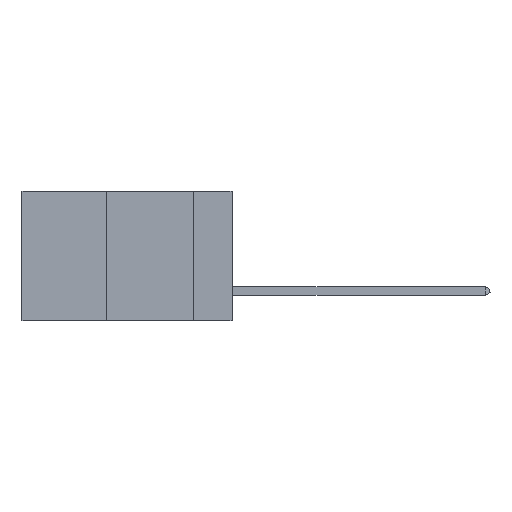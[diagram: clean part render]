
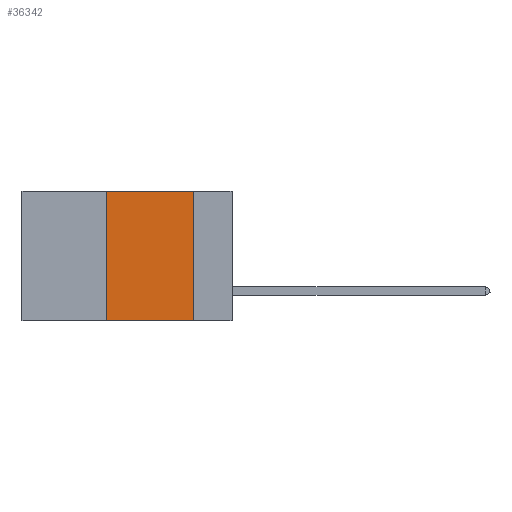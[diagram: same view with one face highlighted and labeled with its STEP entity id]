
A CAD part, left-side view. The second image highlights one B-rep face of the part: STEP entity #36342.
In plain terms, the highlighted planar face has unit normal (-1, 0, 0).
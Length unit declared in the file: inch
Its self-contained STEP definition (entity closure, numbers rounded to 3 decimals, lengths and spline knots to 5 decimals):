
#472 = CARTESIAN_POINT ( 'NONE',  ( 0., 0.36, -0.37 ) ) ;
#2015 = DIRECTION ( 'NONE',  ( 0., -1., 0. ) ) ;
#4391 = ORIENTED_EDGE ( 'NONE', *, *, #30688, .F. ) ;
#5009 = CARTESIAN_POINT ( 'NONE',  ( 0., 0.36, 0. ) ) ;
#8426 = DIRECTION ( 'NONE',  ( 0., 0., 1. ) ) ;
#9119 = ORIENTED_EDGE ( 'NONE', *, *, #25956, .F. ) ;
#10584 = LINE ( 'NONE', #36813, #33721 ) ;
#11051 = CARTESIAN_POINT ( 'NONE',  ( 0., 0.6, 0. ) ) ;
#13673 = AXIS2_PLACEMENT_3D ( 'NONE', #26257, #32345, #29391 ) ;
#14157 = VERTEX_POINT ( 'NONE', #36284 ) ;
#18818 = EDGE_CURVE ( 'NONE', #14157, #27627, #10584, .T. ) ;
#19027 = DIRECTION ( 'NONE',  ( 0., -1., 0. ) ) ;
#19189 = ORIENTED_EDGE ( 'NONE', *, *, #20875, .T. ) ;
#19278 = ORIENTED_EDGE ( 'NONE', *, *, #18818, .F. ) ;
#20875 = EDGE_CURVE ( 'NONE', #21778, #27627, #21733, .T. ) ;
#20915 = LINE ( 'NONE', #11051, #37261 ) ;
#21210 = FACE_OUTER_BOUND ( 'NONE', #39727, .T. ) ;
#21733 = LINE ( 'NONE', #32748, #39582 ) ;
#21778 = VERTEX_POINT ( 'NONE', #472 ) ;
#22618 = VERTEX_POINT ( 'NONE', #5009 ) ;
#25956 = EDGE_CURVE ( 'NONE', #21778, #22618, #35203, .T. ) ;
#26257 = CARTESIAN_POINT ( 'NONE',  ( 0., 0.6, 0. ) ) ;
#27627 = VERTEX_POINT ( 'NONE', #38012 ) ;
#27778 = DIRECTION ( 'NONE',  ( 0., 0., -1. ) ) ;
#29391 = DIRECTION ( 'NONE',  ( 0., 0., -1. ) ) ;
#29536 = PLANE ( 'NONE',  #13673 ) ;
#29552 = CARTESIAN_POINT ( 'NONE',  ( 0., 0.36, 0. ) ) ;
#30688 = EDGE_CURVE ( 'NONE', #22618, #14157, #20915, .T. ) ;
#32345 = DIRECTION ( 'NONE',  ( 1., 0., 0. ) ) ;
#32748 = CARTESIAN_POINT ( 'NONE',  ( 0., 0.6, -0.37 ) ) ;
#33721 = VECTOR ( 'NONE', #27778, 39.37008 ) ;
#33773 = VECTOR ( 'NONE', #8426, 39.37008 ) ;
#35203 = LINE ( 'NONE', #29552, #33773 ) ;
#36284 = CARTESIAN_POINT ( 'NONE',  ( 0., 0.11, 0. ) ) ;
#36342 = ADVANCED_FACE ( 'NONE', ( #21210 ), #29536, .F. ) ;
#36813 = CARTESIAN_POINT ( 'NONE',  ( 0., 0.11, 0. ) ) ;
#37261 = VECTOR ( 'NONE', #2015, 39.37008 ) ;
#38012 = CARTESIAN_POINT ( 'NONE',  ( 0., 0.11, -0.37 ) ) ;
#39582 = VECTOR ( 'NONE', #19027, 39.37008 ) ;
#39727 = EDGE_LOOP ( 'NONE', ( #19278, #4391, #9119, #19189 ) ) ;
